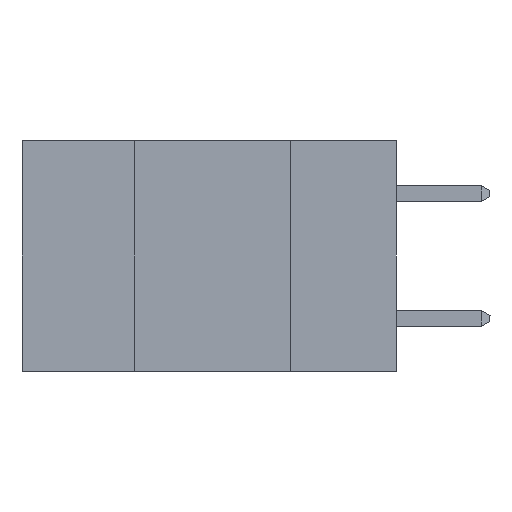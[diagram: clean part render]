
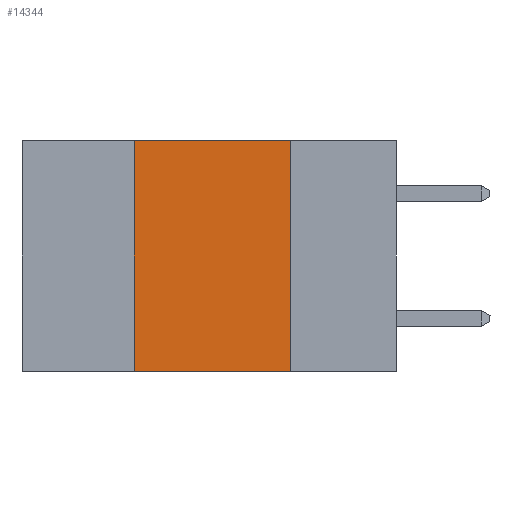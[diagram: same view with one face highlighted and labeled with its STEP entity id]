
A CAD part, left-side view. The second image highlights one B-rep face of the part: STEP entity #14344.
In plain terms, the highlighted planar face has unit normal (-1, 0, 0).
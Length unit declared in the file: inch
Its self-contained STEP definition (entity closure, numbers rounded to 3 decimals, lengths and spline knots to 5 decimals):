
#26 = ORIENTED_EDGE ( 'NONE', *, *, #1810, .F. ) ;
#205 = VECTOR ( 'NONE', #7116, 39.37008 ) ;
#354 = VERTEX_POINT ( 'NONE', #14310 ) ;
#1810 = EDGE_CURVE ( 'NONE', #354, #4558, #3912, .T. ) ;
#1978 = VECTOR ( 'NONE', #8798, 39.37008 ) ;
#3543 = VECTOR ( 'NONE', #9178, 39.37008 ) ;
#3912 = LINE ( 'NONE', #12699, #13418 ) ;
#4122 = ORIENTED_EDGE ( 'NONE', *, *, #10728, .F. ) ;
#4180 = VERTEX_POINT ( 'NONE', #7288 ) ;
#4558 = VERTEX_POINT ( 'NONE', #9674 ) ;
#4686 = EDGE_CURVE ( 'NONE', #4180, #354, #7022, .T. ) ;
#4767 = AXIS2_PLACEMENT_3D ( 'NONE', #14479, #15648, #8434 ) ;
#4794 = FACE_OUTER_BOUND ( 'NONE', #15725, .T. ) ;
#4980 = LINE ( 'NONE', #15982, #1978 ) ;
#5967 = PLANE ( 'NONE',  #4767 ) ;
#6081 = ORIENTED_EDGE ( 'NONE', *, *, #14552, .T. ) ;
#6567 = LINE ( 'NONE', #9863, #3543 ) ;
#6959 = CARTESIAN_POINT ( 'NONE',  ( 0., 0.6, 0. ) ) ;
#7022 = LINE ( 'NONE', #6959, #205 ) ;
#7116 = DIRECTION ( 'NONE',  ( 0., -1., 0. ) ) ;
#7288 = CARTESIAN_POINT ( 'NONE',  ( 0., 0.42, 0. ) ) ;
#8434 = DIRECTION ( 'NONE',  ( 0., 0., -1. ) ) ;
#8798 = DIRECTION ( 'NONE',  ( 0., -1., 0. ) ) ;
#9178 = DIRECTION ( 'NONE',  ( 0., 0., 1. ) ) ;
#9674 = CARTESIAN_POINT ( 'NONE',  ( 0., 0.17, -0.37 ) ) ;
#9863 = CARTESIAN_POINT ( 'NONE',  ( 0., 0.42, -0.37 ) ) ;
#10728 = EDGE_CURVE ( 'NONE', #15445, #4180, #6567, .T. ) ;
#11572 = ORIENTED_EDGE ( 'NONE', *, *, #4686, .F. ) ;
#12649 = DIRECTION ( 'NONE',  ( 0., 0., -1. ) ) ;
#12699 = CARTESIAN_POINT ( 'NONE',  ( 0., 0.17, -0.37 ) ) ;
#13418 = VECTOR ( 'NONE', #12649, 39.37008 ) ;
#13645 = CARTESIAN_POINT ( 'NONE',  ( 0., 0.42, -0.37 ) ) ;
#14310 = CARTESIAN_POINT ( 'NONE',  ( 0., 0.17, 0. ) ) ;
#14344 = ADVANCED_FACE ( 'NONE', ( #4794 ), #5967, .F. ) ;
#14479 = CARTESIAN_POINT ( 'NONE',  ( 0., 0.6, 0. ) ) ;
#14552 = EDGE_CURVE ( 'NONE', #15445, #4558, #4980, .T. ) ;
#15445 = VERTEX_POINT ( 'NONE', #13645 ) ;
#15648 = DIRECTION ( 'NONE',  ( 1., 0., 0. ) ) ;
#15725 = EDGE_LOOP ( 'NONE', ( #26, #11572, #4122, #6081 ) ) ;
#15982 = CARTESIAN_POINT ( 'NONE',  ( 0., 0.6, -0.37 ) ) ;
